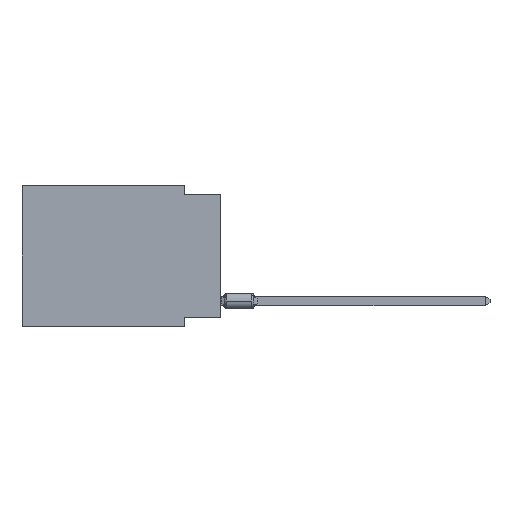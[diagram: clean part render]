
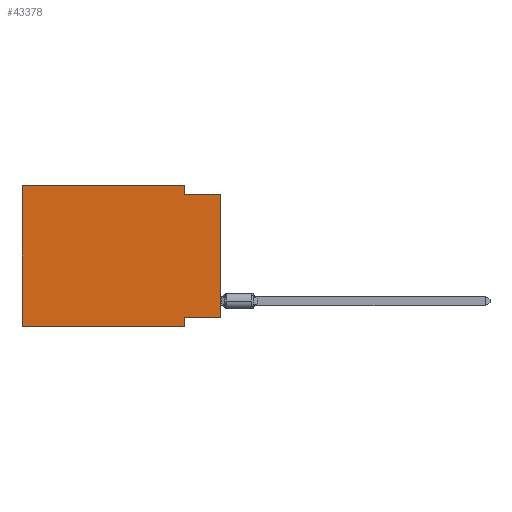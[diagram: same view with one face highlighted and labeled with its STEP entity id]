
A CAD part, left-side view. The second image highlights one B-rep face of the part: STEP entity #43378.
In plain terms, the highlighted planar face has unit normal (-1, 0, 0).
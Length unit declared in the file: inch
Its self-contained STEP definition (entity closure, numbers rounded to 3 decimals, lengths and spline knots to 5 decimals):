
#47 = EDGE_CURVE ( 'NONE', #6093, #22361, #28483, .T. ) ;
#2019 = EDGE_CURVE ( 'NONE', #23789, #21540, #35017, .T. ) ;
#2580 = CARTESIAN_POINT ( 'NONE',  ( 0., 0., -0.025 ) ) ;
#2735 = DIRECTION ( 'NONE',  ( 0., 0., 1. ) ) ;
#2871 = VERTEX_POINT ( 'NONE', #2580 ) ;
#3783 = VECTOR ( 'NONE', #40915, 39.37008 ) ;
#3976 = DIRECTION ( 'NONE',  ( 0., -1., 0. ) ) ;
#4648 = LINE ( 'NONE', #7790, #17335 ) ;
#4717 = CARTESIAN_POINT ( 'NONE',  ( 0., 0.55, -0.39 ) ) ;
#4746 = CARTESIAN_POINT ( 'NONE',  ( 0., 0.1, -0.365 ) ) ;
#5176 = DIRECTION ( 'NONE',  ( 0., 0., -1. ) ) ;
#6093 = VERTEX_POINT ( 'NONE', #16056 ) ;
#6647 = DIRECTION ( 'NONE',  ( 1., 0., 0. ) ) ;
#7764 = VECTOR ( 'NONE', #14824, 39.37008 ) ;
#7790 = CARTESIAN_POINT ( 'NONE',  ( 0., 0., -0.025 ) ) ;
#8732 = VECTOR ( 'NONE', #28718, 39.37008 ) ;
#9629 = CARTESIAN_POINT ( 'NONE',  ( 0., 0.1, -0.39 ) ) ;
#10881 = DIRECTION ( 'NONE',  ( 0., 0., -1. ) ) ;
#12861 = ORIENTED_EDGE ( 'NONE', *, *, #30499, .T. ) ;
#14006 = CARTESIAN_POINT ( 'NONE',  ( 0., 0.55, 0. ) ) ;
#14824 = DIRECTION ( 'NONE',  ( 0., 1., 0. ) ) ;
#15023 = LINE ( 'NONE', #17947, #8732 ) ;
#15241 = CARTESIAN_POINT ( 'NONE',  ( 0., 0.1, 0. ) ) ;
#16056 = CARTESIAN_POINT ( 'NONE',  ( 0., 0.1, 0. ) ) ;
#16389 = EDGE_CURVE ( 'NONE', #26697, #18269, #15023, .T. ) ;
#16877 = VERTEX_POINT ( 'NONE', #28194 ) ;
#17335 = VECTOR ( 'NONE', #3976, 39.37008 ) ;
#17947 = CARTESIAN_POINT ( 'NONE',  ( 0., 0.55, 0. ) ) ;
#18147 = DIRECTION ( 'NONE',  ( 0., -1., 0. ) ) ;
#18269 = VERTEX_POINT ( 'NONE', #27270 ) ;
#19942 = ORIENTED_EDGE ( 'NONE', *, *, #21160, .F. ) ;
#20956 = FACE_OUTER_BOUND ( 'NONE', #27186, .T. ) ;
#21160 = EDGE_CURVE ( 'NONE', #18269, #6093, #38417, .T. ) ;
#21540 = VERTEX_POINT ( 'NONE', #4746 ) ;
#22147 = ORIENTED_EDGE ( 'NONE', *, *, #47, .F. ) ;
#22361 = VERTEX_POINT ( 'NONE', #25948 ) ;
#23789 = VERTEX_POINT ( 'NONE', #26233 ) ;
#24434 = ORIENTED_EDGE ( 'NONE', *, *, #16389, .F. ) ;
#25948 = CARTESIAN_POINT ( 'NONE',  ( 0., 0.1, -0.025 ) ) ;
#26233 = CARTESIAN_POINT ( 'NONE',  ( 0., 0., -0.365 ) ) ;
#26482 = LINE ( 'NONE', #33659, #37147 ) ;
#26697 = VERTEX_POINT ( 'NONE', #4717 ) ;
#27186 = EDGE_LOOP ( 'NONE', ( #12861, #35535, #22147, #19942, #24434, #35394, #33507, #40106 ) ) ;
#27270 = CARTESIAN_POINT ( 'NONE',  ( 0., 0.55, 0. ) ) ;
#28194 = CARTESIAN_POINT ( 'NONE',  ( 0., 0.1, -0.39 ) ) ;
#28460 = CARTESIAN_POINT ( 'NONE',  ( 0., 0.55, -0.39 ) ) ;
#28483 = LINE ( 'NONE', #15241, #37681 ) ;
#28718 = DIRECTION ( 'NONE',  ( 0., 0., 1. ) ) ;
#30025 = VECTOR ( 'NONE', #18147, 39.37008 ) ;
#30499 = EDGE_CURVE ( 'NONE', #23789, #2871, #26482, .T. ) ;
#30815 = EDGE_CURVE ( 'NONE', #26697, #16877, #36295, .T. ) ;
#31670 = CARTESIAN_POINT ( 'NONE',  ( 0., 0., -0.365 ) ) ;
#33507 = ORIENTED_EDGE ( 'NONE', *, *, #35623, .F. ) ;
#33659 = CARTESIAN_POINT ( 'NONE',  ( 0., 0., 0. ) ) ;
#33836 = DIRECTION ( 'NONE',  ( 0., 0., -1. ) ) ;
#34572 = EDGE_CURVE ( 'NONE', #22361, #2871, #4648, .T. ) ;
#35017 = LINE ( 'NONE', #31670, #7764 ) ;
#35394 = ORIENTED_EDGE ( 'NONE', *, *, #30815, .T. ) ;
#35535 = ORIENTED_EDGE ( 'NONE', *, *, #34572, .F. ) ;
#35623 = EDGE_CURVE ( 'NONE', #21540, #16877, #36960, .T. ) ;
#36295 = LINE ( 'NONE', #28460, #30025 ) ;
#36773 = VECTOR ( 'NONE', #33836, 39.37008 ) ;
#36960 = LINE ( 'NONE', #9629, #36773 ) ;
#37115 = AXIS2_PLACEMENT_3D ( 'NONE', #14006, #6647, #10881 ) ;
#37147 = VECTOR ( 'NONE', #2735, 39.37008 ) ;
#37538 = CARTESIAN_POINT ( 'NONE',  ( 0., 0.55, 0. ) ) ;
#37681 = VECTOR ( 'NONE', #5176, 39.37008 ) ;
#38417 = LINE ( 'NONE', #37538, #3783 ) ;
#40106 = ORIENTED_EDGE ( 'NONE', *, *, #2019, .F. ) ;
#40915 = DIRECTION ( 'NONE',  ( 0., -1., 0. ) ) ;
#41352 = PLANE ( 'NONE',  #37115 ) ;
#43378 = ADVANCED_FACE ( 'NONE', ( #20956 ), #41352, .F. ) ;
